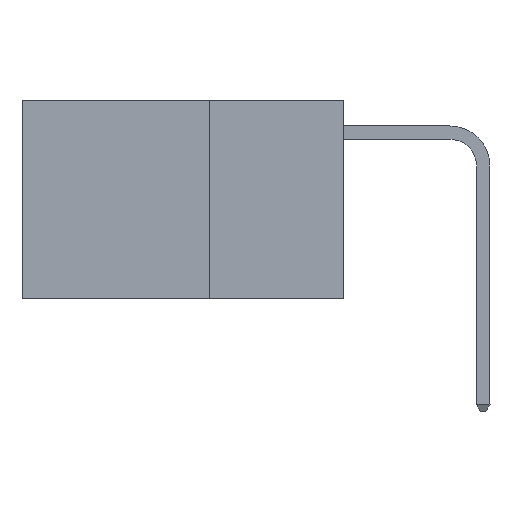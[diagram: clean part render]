
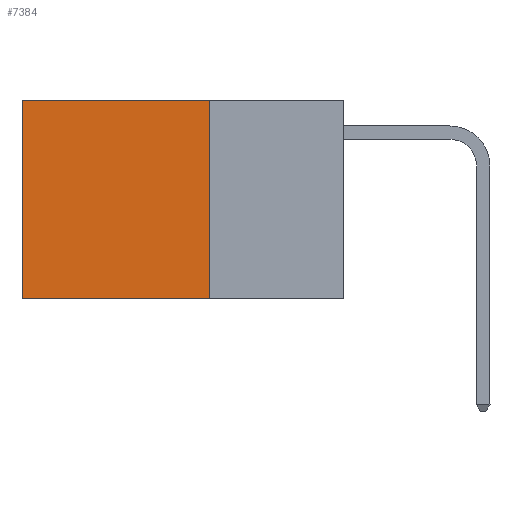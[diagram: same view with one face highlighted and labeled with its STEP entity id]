
A CAD part, left-side view. The second image highlights one B-rep face of the part: STEP entity #7384.
In plain terms, the highlighted planar face has unit normal (-1, 0, 0).
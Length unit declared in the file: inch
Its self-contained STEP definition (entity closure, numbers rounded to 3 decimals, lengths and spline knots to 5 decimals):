
#120 = EDGE_CURVE ( 'NONE', #4149, #5228, #16421, .T. ) ;
#253 = VECTOR ( 'NONE', #2059, 39.37008 ) ;
#383 = EDGE_CURVE ( 'NONE', #4149, #17742, #2039, .T. ) ;
#866 = VECTOR ( 'NONE', #18867, 39.37008 ) ;
#1268 = LINE ( 'NONE', #5965, #8458 ) ;
#2039 = LINE ( 'NONE', #18773, #14769 ) ;
#2059 = DIRECTION ( 'NONE',  ( 0., 0., -1. ) ) ;
#4149 = VERTEX_POINT ( 'NONE', #9223 ) ;
#4152 = PLANE ( 'NONE',  #5820 ) ;
#4221 = CARTESIAN_POINT ( 'NONE',  ( 0.2625, 0.6, -0.37 ) ) ;
#4652 = FACE_OUTER_BOUND ( 'NONE', #12393, .T. ) ;
#5047 = ORIENTED_EDGE ( 'NONE', *, *, #383, .T. ) ;
#5228 = VERTEX_POINT ( 'NONE', #19101 ) ;
#5598 = CARTESIAN_POINT ( 'NONE',  ( 0.2625, 0.6, 0. ) ) ;
#5602 = ORIENTED_EDGE ( 'NONE', *, *, #11958, .F. ) ;
#5820 = AXIS2_PLACEMENT_3D ( 'NONE', #7218, #17721, #8762 ) ;
#5965 = CARTESIAN_POINT ( 'NONE',  ( 0.2625, 0.25, -0.37 ) ) ;
#7218 = CARTESIAN_POINT ( 'NONE',  ( 0.2625, 0.25, 0. ) ) ;
#7384 = ADVANCED_FACE ( 'NONE', ( #4652 ), #4152, .F. ) ;
#7393 = VERTEX_POINT ( 'NONE', #4221 ) ;
#7440 = DIRECTION ( 'NONE',  ( 0., 1., 0. ) ) ;
#8431 = CARTESIAN_POINT ( 'NONE',  ( 0.2625, 0.6, 0. ) ) ;
#8458 = VECTOR ( 'NONE', #7440, 39.37008 ) ;
#8762 = DIRECTION ( 'NONE',  ( 0., 0., -1. ) ) ;
#9223 = CARTESIAN_POINT ( 'NONE',  ( 0.2625, 0.25, 0. ) ) ;
#9651 = DIRECTION ( 'NONE',  ( 0., 1., 0. ) ) ;
#10482 = EDGE_CURVE ( 'NONE', #17742, #7393, #16051, .T. ) ;
#11605 = ORIENTED_EDGE ( 'NONE', *, *, #10482, .T. ) ;
#11958 = EDGE_CURVE ( 'NONE', #5228, #7393, #1268, .T. ) ;
#12143 = ORIENTED_EDGE ( 'NONE', *, *, #120, .F. ) ;
#12393 = EDGE_LOOP ( 'NONE', ( #11605, #5602, #12143, #5047 ) ) ;
#13086 = CARTESIAN_POINT ( 'NONE',  ( 0.2625, 0.25, 0. ) ) ;
#14769 = VECTOR ( 'NONE', #9651, 39.37008 ) ;
#16051 = LINE ( 'NONE', #8431, #866 ) ;
#16421 = LINE ( 'NONE', #13086, #253 ) ;
#17721 = DIRECTION ( 'NONE',  ( 1., 0., 0. ) ) ;
#17742 = VERTEX_POINT ( 'NONE', #5598 ) ;
#18773 = CARTESIAN_POINT ( 'NONE',  ( 0.2625, 0.25, 0. ) ) ;
#18867 = DIRECTION ( 'NONE',  ( 0., 0., -1. ) ) ;
#19101 = CARTESIAN_POINT ( 'NONE',  ( 0.2625, 0.25, -0.37 ) ) ;
